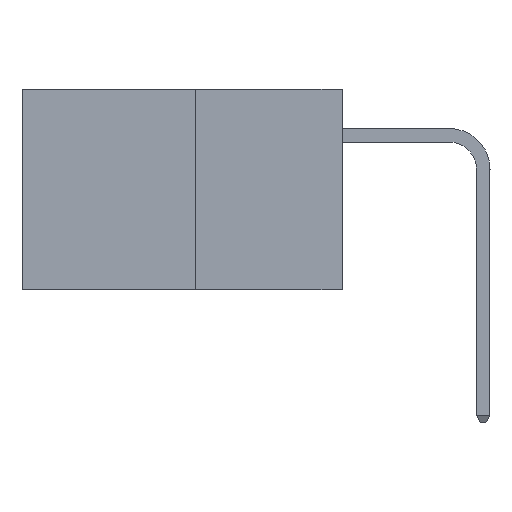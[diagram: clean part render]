
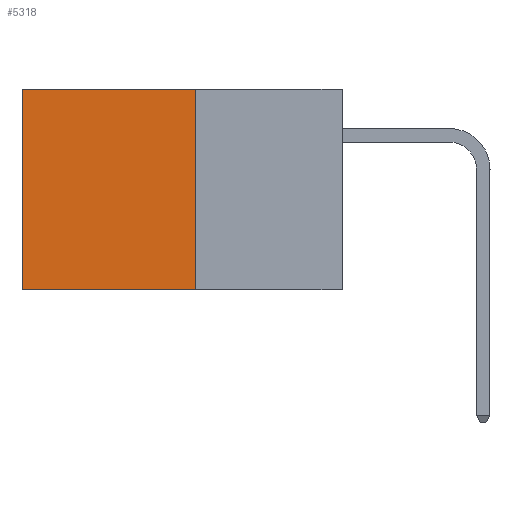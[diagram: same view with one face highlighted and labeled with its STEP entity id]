
A CAD part, left-side view. The second image highlights one B-rep face of the part: STEP entity #5318.
In plain terms, the highlighted planar face has unit normal (-1, 0, 0).
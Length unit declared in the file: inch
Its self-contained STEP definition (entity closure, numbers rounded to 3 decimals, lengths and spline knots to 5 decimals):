
#1346 = CARTESIAN_POINT ( 'NONE',  ( 0.277, 0.59, -0.37 ) ) ;
#1370 = LINE ( 'NONE', #10821, #9799 ) ;
#1662 = FACE_OUTER_BOUND ( 'NONE', #6368, .T. ) ;
#1723 = ORIENTED_EDGE ( 'NONE', *, *, #4614, .F. ) ;
#1750 = DIRECTION ( 'NONE',  ( 0., 0., -1. ) ) ;
#2084 = VECTOR ( 'NONE', #9818, 39.37008 ) ;
#2262 = AXIS2_PLACEMENT_3D ( 'NONE', #6070, #6892, #1750 ) ;
#2265 = VECTOR ( 'NONE', #5150, 39.37008 ) ;
#2284 = VERTEX_POINT ( 'NONE', #4082 ) ;
#2742 = CARTESIAN_POINT ( 'NONE',  ( 0.277, 0.59, 0. ) ) ;
#3444 = CARTESIAN_POINT ( 'NONE',  ( 0.277, 0.59, -0.37 ) ) ;
#3462 = EDGE_CURVE ( 'NONE', #2284, #3687, #10628, .T. ) ;
#3687 = VERTEX_POINT ( 'NONE', #2742 ) ;
#3937 = DIRECTION ( 'NONE',  ( 0., 0., -1. ) ) ;
#3947 = VERTEX_POINT ( 'NONE', #3444 ) ;
#4082 = CARTESIAN_POINT ( 'NONE',  ( 0.277, 0.27, 0. ) ) ;
#4121 = LINE ( 'NONE', #9830, #2084 ) ;
#4614 = EDGE_CURVE ( 'NONE', #9383, #3947, #4121, .T. ) ;
#5150 = DIRECTION ( 'NONE',  ( 0., 1., 0. ) ) ;
#5157 = CARTESIAN_POINT ( 'NONE',  ( 0.277, 0.27, 0. ) ) ;
#5315 = ORIENTED_EDGE ( 'NONE', *, *, #3462, .T. ) ;
#5318 = ADVANCED_FACE ( 'NONE', ( #1662 ), #6458, .F. ) ;
#6070 = CARTESIAN_POINT ( 'NONE',  ( 0.277, 0.27, -0.37 ) ) ;
#6368 = EDGE_LOOP ( 'NONE', ( #9151, #1723, #10787, #5315 ) ) ;
#6458 = PLANE ( 'NONE',  #2262 ) ;
#6892 = DIRECTION ( 'NONE',  ( 1., 0., 0. ) ) ;
#7904 = VECTOR ( 'NONE', #3937, 39.37008 ) ;
#8138 = EDGE_CURVE ( 'NONE', #2284, #9383, #1370, .T. ) ;
#8156 = LINE ( 'NONE', #1346, #7904 ) ;
#9151 = ORIENTED_EDGE ( 'NONE', *, *, #10914, .T. ) ;
#9253 = CARTESIAN_POINT ( 'NONE',  ( 0.277, 0.27, -0.37 ) ) ;
#9383 = VERTEX_POINT ( 'NONE', #9253 ) ;
#9799 = VECTOR ( 'NONE', #9980, 39.37008 ) ;
#9818 = DIRECTION ( 'NONE',  ( 0., 1., 0. ) ) ;
#9830 = CARTESIAN_POINT ( 'NONE',  ( 0.277, 0.27, -0.37 ) ) ;
#9980 = DIRECTION ( 'NONE',  ( 0., 0., -1. ) ) ;
#10628 = LINE ( 'NONE', #5157, #2265 ) ;
#10787 = ORIENTED_EDGE ( 'NONE', *, *, #8138, .F. ) ;
#10821 = CARTESIAN_POINT ( 'NONE',  ( 0.277, 0.27, -0.37 ) ) ;
#10914 = EDGE_CURVE ( 'NONE', #3687, #3947, #8156, .T. ) ;
